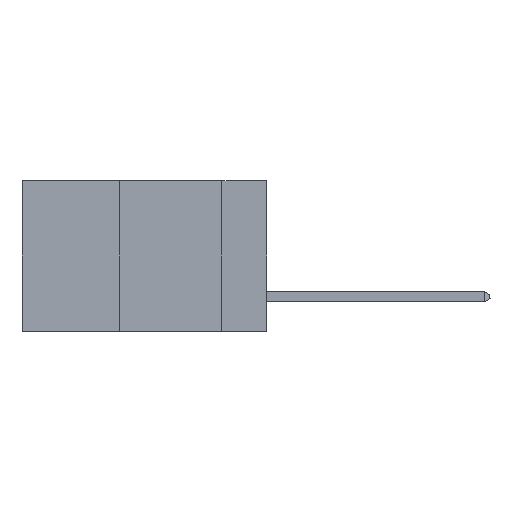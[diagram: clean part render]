
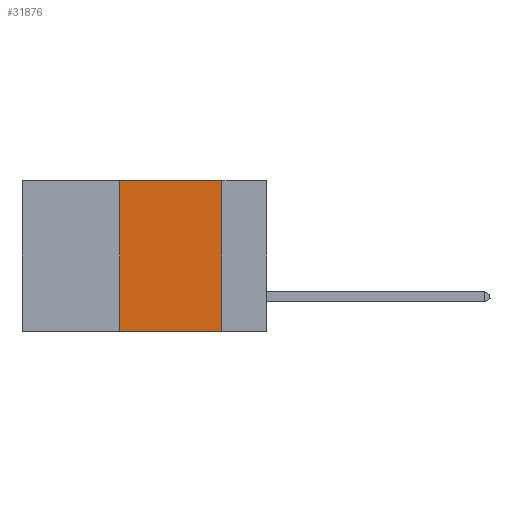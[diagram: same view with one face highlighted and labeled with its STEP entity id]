
A CAD part, left-side view. The second image highlights one B-rep face of the part: STEP entity #31876.
In plain terms, the highlighted planar face has unit normal (-1, 0, 0).
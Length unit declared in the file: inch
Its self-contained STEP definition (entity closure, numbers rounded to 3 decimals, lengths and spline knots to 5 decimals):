
#324 = ORIENTED_EDGE ( 'NONE', *, *, #12040, .F. ) ;
#3602 = DIRECTION ( 'NONE',  ( 0., 0., 1. ) ) ;
#4571 = ORIENTED_EDGE ( 'NONE', *, *, #10902, .T. ) ;
#4575 = VECTOR ( 'NONE', #28174, 39.37008 ) ;
#9018 = ORIENTED_EDGE ( 'NONE', *, *, #40182, .F. ) ;
#10816 = ORIENTED_EDGE ( 'NONE', *, *, #44541, .F. ) ;
#10902 = EDGE_CURVE ( 'NONE', #36180, #24700, #30520, .T. ) ;
#12040 = EDGE_CURVE ( 'NONE', #33033, #24700, #49637, .T. ) ;
#14977 = DIRECTION ( 'NONE',  ( 0., 0., -1. ) ) ;
#15234 = CARTESIAN_POINT ( 'NONE',  ( 0., 0.11, 0. ) ) ;
#16786 = CARTESIAN_POINT ( 'NONE',  ( 0., 0.11, 0. ) ) ;
#18743 = VERTEX_POINT ( 'NONE', #41123 ) ;
#24004 = LINE ( 'NONE', #43191, #48014 ) ;
#24700 = VERTEX_POINT ( 'NONE', #49621 ) ;
#27949 = VECTOR ( 'NONE', #41862, 39.37008 ) ;
#28174 = DIRECTION ( 'NONE',  ( 0., -1., 0. ) ) ;
#29000 = AXIS2_PLACEMENT_3D ( 'NONE', #34264, #30450, #14977 ) ;
#30001 = CARTESIAN_POINT ( 'NONE',  ( 0., 0.36, 0. ) ) ;
#30450 = DIRECTION ( 'NONE',  ( 1., 0., 0. ) ) ;
#30520 = LINE ( 'NONE', #47568, #4575 ) ;
#30916 = PLANE ( 'NONE',  #29000 ) ;
#31876 = ADVANCED_FACE ( 'NONE', ( #39431 ), #30916, .F. ) ;
#33033 = VERTEX_POINT ( 'NONE', #16786 ) ;
#34264 = CARTESIAN_POINT ( 'NONE',  ( 0., 0.6, 0. ) ) ;
#35298 = EDGE_LOOP ( 'NONE', ( #324, #9018, #10816, #4571 ) ) ;
#36160 = DIRECTION ( 'NONE',  ( 0., -1., 0. ) ) ;
#36180 = VERTEX_POINT ( 'NONE', #48246 ) ;
#39431 = FACE_OUTER_BOUND ( 'NONE', #35298, .T. ) ;
#40182 = EDGE_CURVE ( 'NONE', #18743, #33033, #24004, .T. ) ;
#40348 = VECTOR ( 'NONE', #3602, 39.37008 ) ;
#41123 = CARTESIAN_POINT ( 'NONE',  ( 0., 0.36, 0. ) ) ;
#41862 = DIRECTION ( 'NONE',  ( 0., 0., -1. ) ) ;
#43191 = CARTESIAN_POINT ( 'NONE',  ( 0., 0.6, 0. ) ) ;
#44541 = EDGE_CURVE ( 'NONE', #36180, #18743, #46403, .T. ) ;
#46403 = LINE ( 'NONE', #30001, #40348 ) ;
#47568 = CARTESIAN_POINT ( 'NONE',  ( 0., 0.6, -0.37 ) ) ;
#48014 = VECTOR ( 'NONE', #36160, 39.37008 ) ;
#48246 = CARTESIAN_POINT ( 'NONE',  ( 0., 0.36, -0.37 ) ) ;
#49621 = CARTESIAN_POINT ( 'NONE',  ( 0., 0.11, -0.37 ) ) ;
#49637 = LINE ( 'NONE', #15234, #27949 ) ;
